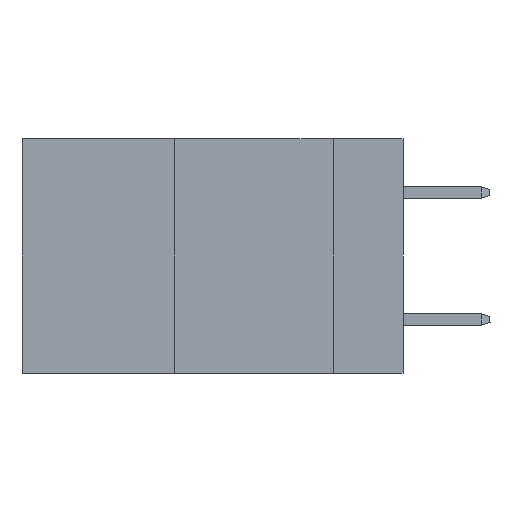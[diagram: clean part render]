
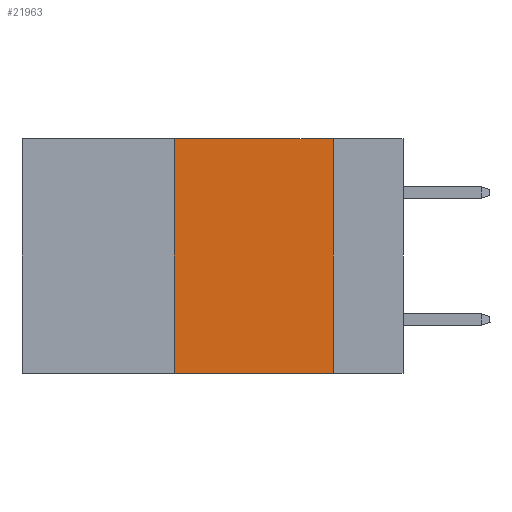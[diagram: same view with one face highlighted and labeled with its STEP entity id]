
A CAD part, left-side view. The second image highlights one B-rep face of the part: STEP entity #21963.
In plain terms, the highlighted planar face has unit normal (-1, 0, 0).
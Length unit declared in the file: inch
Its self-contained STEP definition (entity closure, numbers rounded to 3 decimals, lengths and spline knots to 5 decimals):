
#640 = EDGE_CURVE ( 'NONE', #20306, #14214, #22432, .T. ) ;
#895 = FACE_OUTER_BOUND ( 'NONE', #2414, .T. ) ;
#2193 = LINE ( 'NONE', #24480, #8561 ) ;
#2414 = EDGE_LOOP ( 'NONE', ( #5841, #24209, #7784, #15009 ) ) ;
#2742 = CARTESIAN_POINT ( 'NONE',  ( 0., 0.6, 0. ) ) ;
#4370 = EDGE_CURVE ( 'NONE', #17657, #20306, #6254, .T. ) ;
#4557 = DIRECTION ( 'NONE',  ( 0., -1., 0. ) ) ;
#5841 = ORIENTED_EDGE ( 'NONE', *, *, #640, .F. ) ;
#6121 = VECTOR ( 'NONE', #13515, 39.37008 ) ;
#6254 = LINE ( 'NONE', #22240, #21097 ) ;
#6688 = DIRECTION ( 'NONE',  ( 0., 0., -1. ) ) ;
#6828 = EDGE_CURVE ( 'NONE', #16649, #14214, #2193, .T. ) ;
#7366 = CARTESIAN_POINT ( 'NONE',  ( 0., 0.36, 0. ) ) ;
#7409 = CARTESIAN_POINT ( 'NONE',  ( 0., 0.11, -0.37 ) ) ;
#7784 = ORIENTED_EDGE ( 'NONE', *, *, #10511, .F. ) ;
#7788 = CARTESIAN_POINT ( 'NONE',  ( 0., 0.36, 0. ) ) ;
#8458 = VECTOR ( 'NONE', #19972, 39.37008 ) ;
#8561 = VECTOR ( 'NONE', #4557, 39.37008 ) ;
#10511 = EDGE_CURVE ( 'NONE', #16649, #17657, #25331, .T. ) ;
#12706 = PLANE ( 'NONE',  #16396 ) ;
#13515 = DIRECTION ( 'NONE',  ( 0., 0., 1. ) ) ;
#14214 = VERTEX_POINT ( 'NONE', #7409 ) ;
#15009 = ORIENTED_EDGE ( 'NONE', *, *, #6828, .T. ) ;
#16396 = AXIS2_PLACEMENT_3D ( 'NONE', #2742, #20982, #6688 ) ;
#16649 = VERTEX_POINT ( 'NONE', #18888 ) ;
#17657 = VERTEX_POINT ( 'NONE', #7788 ) ;
#18888 = CARTESIAN_POINT ( 'NONE',  ( 0., 0.36, -0.37 ) ) ;
#19909 = DIRECTION ( 'NONE',  ( 0., -1., 0. ) ) ;
#19972 = DIRECTION ( 'NONE',  ( 0., 0., -1. ) ) ;
#20306 = VERTEX_POINT ( 'NONE', #25152 ) ;
#20982 = DIRECTION ( 'NONE',  ( 1., 0., 0. ) ) ;
#21097 = VECTOR ( 'NONE', #19909, 39.37008 ) ;
#21963 = ADVANCED_FACE ( 'NONE', ( #895 ), #12706, .F. ) ;
#22240 = CARTESIAN_POINT ( 'NONE',  ( 0., 0.6, 0. ) ) ;
#22432 = LINE ( 'NONE', #23987, #8458 ) ;
#23987 = CARTESIAN_POINT ( 'NONE',  ( 0., 0.11, 0. ) ) ;
#24209 = ORIENTED_EDGE ( 'NONE', *, *, #4370, .F. ) ;
#24480 = CARTESIAN_POINT ( 'NONE',  ( 0., 0.6, -0.37 ) ) ;
#25152 = CARTESIAN_POINT ( 'NONE',  ( 0., 0.11, 0. ) ) ;
#25331 = LINE ( 'NONE', #7366, #6121 ) ;
